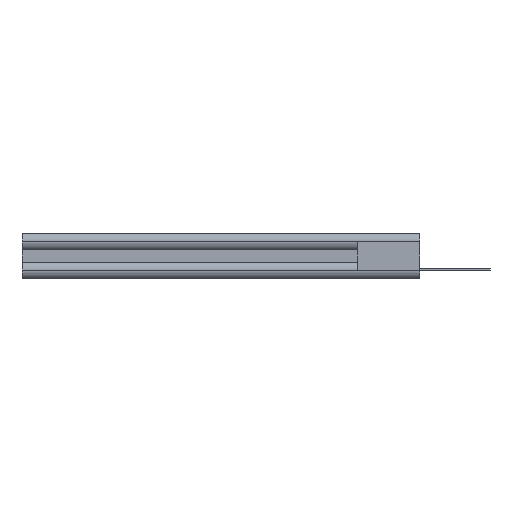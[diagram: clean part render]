
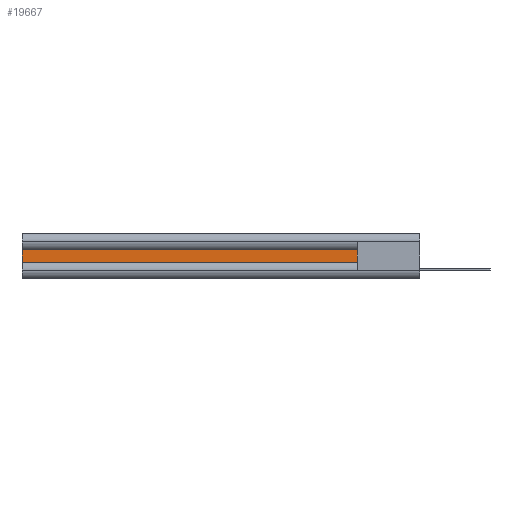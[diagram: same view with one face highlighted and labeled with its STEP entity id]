
A CAD part, left-side view. The second image highlights one B-rep face of the part: STEP entity #19667.
In plain terms, the highlighted planar face has unit normal (-1, 0, 0).
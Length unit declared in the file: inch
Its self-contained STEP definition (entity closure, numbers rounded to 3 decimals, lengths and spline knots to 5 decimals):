
#1120 = VECTOR ( 'NONE', #18828, 39.37008 ) ;
#2129 = ORIENTED_EDGE ( 'NONE', *, *, #9038, .F. ) ;
#2195 = DIRECTION ( 'NONE',  ( 1., 0., 0. ) ) ;
#4172 = LINE ( 'NONE', #14243, #21730 ) ;
#5260 = CARTESIAN_POINT ( 'NONE',  ( 0.044, 3., 0.0465 ) ) ;
#6041 = DIRECTION ( 'NONE',  ( 0., 1., 0. ) ) ;
#6805 = LINE ( 'NONE', #12848, #19255 ) ;
#8285 = VERTEX_POINT ( 'NONE', #19329 ) ;
#8544 = DIRECTION ( 'NONE',  ( 0., 1., 0. ) ) ;
#8699 = CARTESIAN_POINT ( 'NONE',  ( 0.044, 3., -0.0465 ) ) ;
#9038 = EDGE_CURVE ( 'NONE', #12101, #11306, #6805, .T. ) ;
#9200 = DIRECTION ( 'NONE',  ( 0., 0., -1. ) ) ;
#10842 = PLANE ( 'NONE',  #16885 ) ;
#10989 = FACE_OUTER_BOUND ( 'NONE', #18805, .T. ) ;
#11306 = VERTEX_POINT ( 'NONE', #14263 ) ;
#12101 = VERTEX_POINT ( 'NONE', #21364 ) ;
#12558 = CARTESIAN_POINT ( 'NONE',  ( 0.044, 0.37012, -0.0465 ) ) ;
#12848 = CARTESIAN_POINT ( 'NONE',  ( 0.044, 0.37012, -0.0465 ) ) ;
#14243 = CARTESIAN_POINT ( 'NONE',  ( 0.044, 0.473, -0.0465 ) ) ;
#14252 = DIRECTION ( 'NONE',  ( 0., 0., -1. ) ) ;
#14263 = CARTESIAN_POINT ( 'NONE',  ( 0.044, 3., -0.0465 ) ) ;
#14882 = LINE ( 'NONE', #8699, #1120 ) ;
#15695 = EDGE_CURVE ( 'NONE', #18964, #11306, #14882, .T. ) ;
#16885 = AXIS2_PLACEMENT_3D ( 'NONE', #12558, #2195, #14252 ) ;
#18805 = EDGE_LOOP ( 'NONE', ( #21448, #22240, #2129, #18841 ) ) ;
#18828 = DIRECTION ( 'NONE',  ( 0., 0., -1. ) ) ;
#18841 = ORIENTED_EDGE ( 'NONE', *, *, #20858, .F. ) ;
#18964 = VERTEX_POINT ( 'NONE', #5260 ) ;
#19166 = VECTOR ( 'NONE', #8544, 39.37008 ) ;
#19255 = VECTOR ( 'NONE', #6041, 39.37008 ) ;
#19329 = CARTESIAN_POINT ( 'NONE',  ( 0.044, 0.473, 0.0465 ) ) ;
#19480 = EDGE_CURVE ( 'NONE', #8285, #18964, #20235, .T. ) ;
#19667 = ADVANCED_FACE ( 'NONE', ( #10989 ), #10842, .F. ) ;
#20235 = LINE ( 'NONE', #20441, #19166 ) ;
#20441 = CARTESIAN_POINT ( 'NONE',  ( 0.044, 0.37012, 0.0465 ) ) ;
#20858 = EDGE_CURVE ( 'NONE', #8285, #12101, #4172, .T. ) ;
#21364 = CARTESIAN_POINT ( 'NONE',  ( 0.044, 0.473, -0.0465 ) ) ;
#21448 = ORIENTED_EDGE ( 'NONE', *, *, #19480, .T. ) ;
#21730 = VECTOR ( 'NONE', #9200, 39.37008 ) ;
#22240 = ORIENTED_EDGE ( 'NONE', *, *, #15695, .T. ) ;
